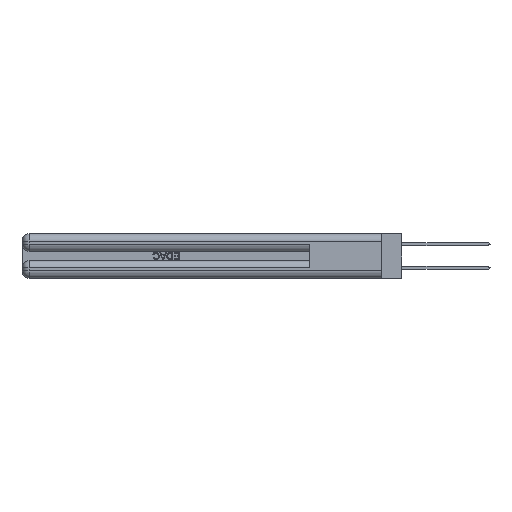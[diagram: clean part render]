
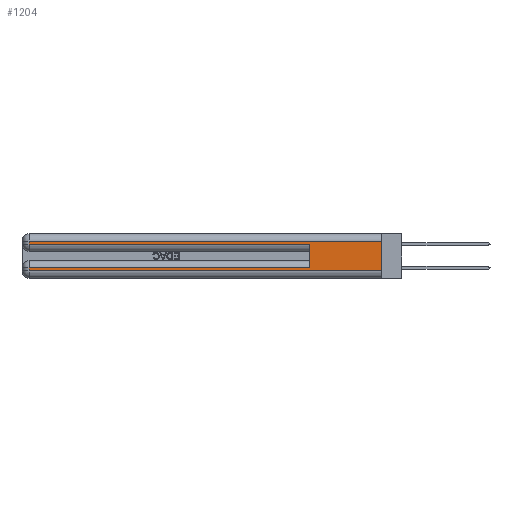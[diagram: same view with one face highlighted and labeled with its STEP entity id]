
A CAD part, left-side view. The second image highlights one B-rep face of the part: STEP entity #1204.
In plain terms, the highlighted planar face has unit normal (-1, 0, 0).
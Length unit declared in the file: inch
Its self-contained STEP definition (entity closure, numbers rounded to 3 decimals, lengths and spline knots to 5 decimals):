
#287 = VECTOR ( 'NONE', #12833, 39.37008 ) ;
#1204 = ADVANCED_FACE ( 'NONE', ( #7654 ), #15799, .F. ) ;
#1218 = LINE ( 'NONE', #43228, #27815 ) ;
#1256 = CARTESIAN_POINT ( 'NONE',  ( 0., 0., 0.06 ) ) ;
#1838 = DIRECTION ( 'NONE',  ( 0., 0., -1. ) ) ;
#2746 = VECTOR ( 'NONE', #30688, 39.37008 ) ;
#3441 = CARTESIAN_POINT ( 'NONE',  ( 0., 0.6, 0.085 ) ) ;
#3574 = DIRECTION ( 'NONE',  ( 1., 0., 0. ) ) ;
#4545 = EDGE_CURVE ( 'NONE', #37799, #39113, #1218, .T. ) ;
#4875 = ORIENTED_EDGE ( 'NONE', *, *, #9565, .F. ) ;
#6569 = CARTESIAN_POINT ( 'NONE',  ( 0., 0., 0.085 ) ) ;
#7654 = FACE_OUTER_BOUND ( 'NONE', #34008, .T. ) ;
#8452 = ORIENTED_EDGE ( 'NONE', *, *, #4545, .T. ) ;
#9099 = DIRECTION ( 'NONE',  ( 0., 0., -1. ) ) ;
#9565 = EDGE_CURVE ( 'NONE', #26014, #35403, #13211, .T. ) ;
#9663 = CARTESIAN_POINT ( 'NONE',  ( 0., 0.6, 0.285 ) ) ;
#9759 = LINE ( 'NONE', #40126, #287 ) ;
#10062 = VECTOR ( 'NONE', #27826, 39.37008 ) ;
#11162 = LINE ( 'NONE', #24383, #10062 ) ;
#12821 = VECTOR ( 'NONE', #9099, 39.37008 ) ;
#12833 = DIRECTION ( 'NONE',  ( 0., 0., 1. ) ) ;
#12931 = ORIENTED_EDGE ( 'NONE', *, *, #36188, .T. ) ;
#13211 = LINE ( 'NONE', #44334, #2746 ) ;
#14668 = EDGE_CURVE ( 'NONE', #40590, #35403, #44498, .T. ) ;
#15799 = PLANE ( 'NONE',  #32247 ) ;
#16285 = EDGE_CURVE ( 'NONE', #39113, #21992, #11162, .T. ) ;
#18041 = VERTEX_POINT ( 'NONE', #3441 ) ;
#18835 = VECTOR ( 'NONE', #30732, 39.37008 ) ;
#19403 = CARTESIAN_POINT ( 'NONE',  ( 0., 2.94, 0.37 ) ) ;
#19886 = LINE ( 'NONE', #6569, #18835 ) ;
#19917 = ORIENTED_EDGE ( 'NONE', *, *, #31603, .T. ) ;
#21975 = LINE ( 'NONE', #19403, #12821 ) ;
#21992 = VERTEX_POINT ( 'NONE', #9663 ) ;
#23606 = ORIENTED_EDGE ( 'NONE', *, *, #41561, .F. ) ;
#24349 = CARTESIAN_POINT ( 'NONE',  ( 0., 0., 0.37 ) ) ;
#24383 = CARTESIAN_POINT ( 'NONE',  ( 0., 0., 0.285 ) ) ;
#25175 = VECTOR ( 'NONE', #43854, 39.37008 ) ;
#26014 = VERTEX_POINT ( 'NONE', #32684 ) ;
#27786 = DIRECTION ( 'NONE',  ( 0., 0., -1. ) ) ;
#27815 = VECTOR ( 'NONE', #1838, 39.37008 ) ;
#27826 = DIRECTION ( 'NONE',  ( 0., -1., 0. ) ) ;
#28990 = ORIENTED_EDGE ( 'NONE', *, *, #35520, .T. ) ;
#30688 = DIRECTION ( 'NONE',  ( 0., 0., -1. ) ) ;
#30732 = DIRECTION ( 'NONE',  ( 0., 1., 0. ) ) ;
#31603 = EDGE_CURVE ( 'NONE', #18041, #36707, #19886, .T. ) ;
#32247 = AXIS2_PLACEMENT_3D ( 'NONE', #24349, #3574, #27786 ) ;
#32301 = CARTESIAN_POINT ( 'NONE',  ( 0., 2.94, 0.31 ) ) ;
#32684 = CARTESIAN_POINT ( 'NONE',  ( 0., 0., 0.31 ) ) ;
#33061 = CARTESIAN_POINT ( 'NONE',  ( 0., 0., 0.31 ) ) ;
#33296 = VECTOR ( 'NONE', #36497, 39.37008 ) ;
#33725 = CARTESIAN_POINT ( 'NONE',  ( 0., 2.94, 0.085 ) ) ;
#34008 = EDGE_LOOP ( 'NONE', ( #4875, #28990, #8452, #43083, #23606, #19917, #12931, #40298 ) ) ;
#35403 = VERTEX_POINT ( 'NONE', #1256 ) ;
#35460 = LINE ( 'NONE', #33061, #33296 ) ;
#35520 = EDGE_CURVE ( 'NONE', #26014, #37799, #35460, .T. ) ;
#36188 = EDGE_CURVE ( 'NONE', #36707, #40590, #21975, .T. ) ;
#36497 = DIRECTION ( 'NONE',  ( 0., 1., 0. ) ) ;
#36707 = VERTEX_POINT ( 'NONE', #33725 ) ;
#36959 = CARTESIAN_POINT ( 'NONE',  ( 0., 0., 0.06 ) ) ;
#37799 = VERTEX_POINT ( 'NONE', #32301 ) ;
#38416 = CARTESIAN_POINT ( 'NONE',  ( 0., 2.94, 0.06 ) ) ;
#39113 = VERTEX_POINT ( 'NONE', #43555 ) ;
#40126 = CARTESIAN_POINT ( 'NONE',  ( 0., 0.6, 0.145 ) ) ;
#40298 = ORIENTED_EDGE ( 'NONE', *, *, #14668, .T. ) ;
#40590 = VERTEX_POINT ( 'NONE', #38416 ) ;
#41561 = EDGE_CURVE ( 'NONE', #18041, #21992, #9759, .T. ) ;
#43083 = ORIENTED_EDGE ( 'NONE', *, *, #16285, .T. ) ;
#43228 = CARTESIAN_POINT ( 'NONE',  ( 0., 2.94, 0.37 ) ) ;
#43555 = CARTESIAN_POINT ( 'NONE',  ( 0., 2.94, 0.285 ) ) ;
#43854 = DIRECTION ( 'NONE',  ( 0., -1., 0. ) ) ;
#44334 = CARTESIAN_POINT ( 'NONE',  ( 0., 0., 0.37 ) ) ;
#44498 = LINE ( 'NONE', #36959, #25175 ) ;
